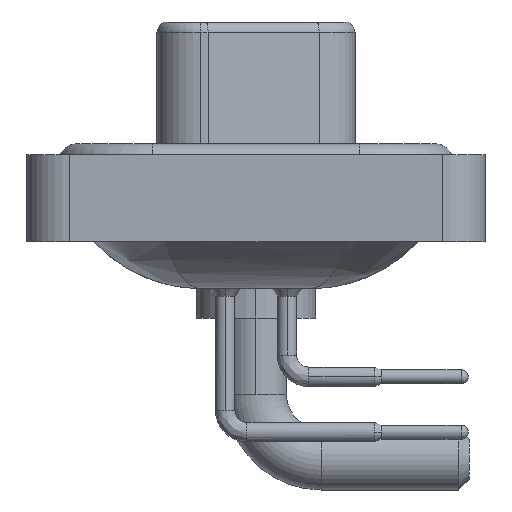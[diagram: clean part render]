
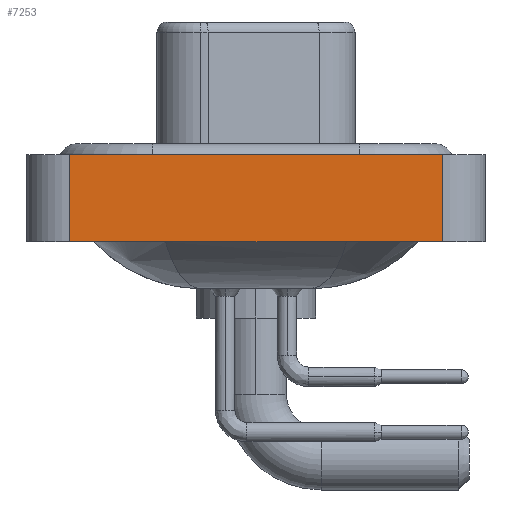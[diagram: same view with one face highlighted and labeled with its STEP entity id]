
A CAD part, left-side view. The second image highlights one B-rep face of the part: STEP entity #7253.
In plain terms, the highlighted planar face has unit normal (-1, 0, 0).
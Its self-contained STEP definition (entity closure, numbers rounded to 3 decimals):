
#443 = DIRECTION ( 'NONE',  ( 0., 0., 1. ) ) ;
#601 = LINE ( 'NONE', #16371, #18810 ) ;
#751 = ORIENTED_EDGE ( 'NONE', *, *, #15708, .F. ) ;
#1234 = CARTESIAN_POINT ( 'NONE',  ( -7.3, -8.55, -3.6 ) ) ;
#3510 = EDGE_LOOP ( 'NONE', ( #25493, #20156, #751, #17996 ) ) ;
#4047 = EDGE_CURVE ( 'NONE', #25336, #21676, #10883, .T. ) ;
#4325 = VECTOR ( 'NONE', #18631, 1000. ) ;
#4622 = CARTESIAN_POINT ( 'NONE',  ( -7.3, 8.55, -3.6 ) ) ;
#4730 = EDGE_CURVE ( 'NONE', #18935, #21676, #22476, .T. ) ;
#6858 = VECTOR ( 'NONE', #24573, 1000. ) ;
#7253 = ADVANCED_FACE ( 'NONE', ( #25241 ), #7657, .T. ) ;
#7657 = PLANE ( 'NONE',  #21605 ) ;
#8609 = DIRECTION ( 'NONE',  ( 0., -1., 0. ) ) ;
#8802 = VECTOR ( 'NONE', #443, 1000. ) ;
#10847 = EDGE_CURVE ( 'NONE', #15161, #18935, #601, .T. ) ;
#10883 = LINE ( 'NONE', #18874, #4325 ) ;
#11022 = CARTESIAN_POINT ( 'NONE',  ( -7.3, -8.55, -3.6 ) ) ;
#13467 = DIRECTION ( 'NONE',  ( -1., 0., 0. ) ) ;
#15161 = VERTEX_POINT ( 'NONE', #24237 ) ;
#15708 = EDGE_CURVE ( 'NONE', #15161, #25336, #22619, .T. ) ;
#16371 = CARTESIAN_POINT ( 'NONE',  ( -7.3, -8.55, -3.6 ) ) ;
#17996 = ORIENTED_EDGE ( 'NONE', *, *, #10847, .T. ) ;
#18631 = DIRECTION ( 'NONE',  ( 0., -1., 0. ) ) ;
#18810 = VECTOR ( 'NONE', #8609, 1000. ) ;
#18874 = CARTESIAN_POINT ( 'NONE',  ( -7.3, -8.55, 0.4 ) ) ;
#18935 = VERTEX_POINT ( 'NONE', #11022 ) ;
#20156 = ORIENTED_EDGE ( 'NONE', *, *, #4047, .F. ) ;
#20899 = CARTESIAN_POINT ( 'NONE',  ( -7.3, -8.55, -3.6 ) ) ;
#21252 = CARTESIAN_POINT ( 'NONE',  ( -7.3, -8.55, 0.4 ) ) ;
#21605 = AXIS2_PLACEMENT_3D ( 'NONE', #1234, #13467, #25501 ) ;
#21676 = VERTEX_POINT ( 'NONE', #21252 ) ;
#22476 = LINE ( 'NONE', #20899, #6858 ) ;
#22619 = LINE ( 'NONE', #4622, #8802 ) ;
#24105 = CARTESIAN_POINT ( 'NONE',  ( -7.3, 8.55, 0.4 ) ) ;
#24237 = CARTESIAN_POINT ( 'NONE',  ( -7.3, 8.55, -3.6 ) ) ;
#24573 = DIRECTION ( 'NONE',  ( 0., 0., 1. ) ) ;
#25241 = FACE_OUTER_BOUND ( 'NONE', #3510, .T. ) ;
#25336 = VERTEX_POINT ( 'NONE', #24105 ) ;
#25493 = ORIENTED_EDGE ( 'NONE', *, *, #4730, .T. ) ;
#25501 = DIRECTION ( 'NONE',  ( 0., 0., 1. ) ) ;
